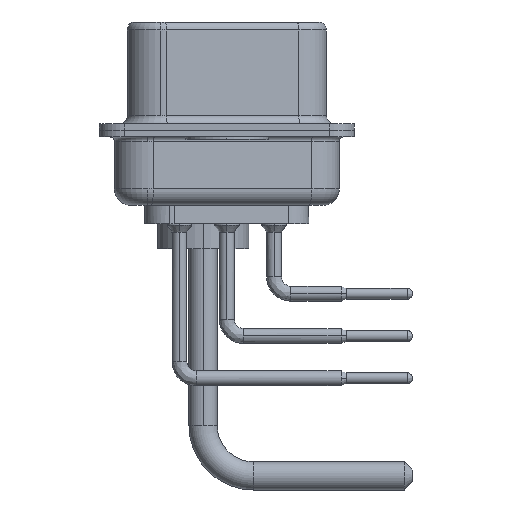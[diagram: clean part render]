
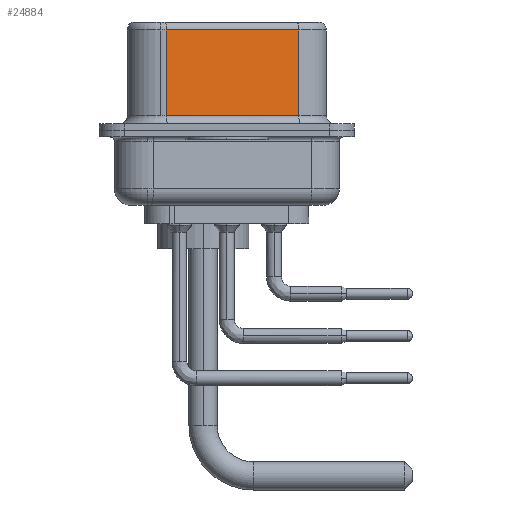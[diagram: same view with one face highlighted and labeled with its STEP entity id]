
A CAD part, left-side view. The second image highlights one B-rep face of the part: STEP entity #24884.
In plain terms, the highlighted planar face has unit normal (-0.985, -0.174, 0).
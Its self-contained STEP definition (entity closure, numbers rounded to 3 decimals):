
#595 = CARTESIAN_POINT ( 'NONE',  ( 5.132, -4.322, 0.9 ) ) ;
#797 = ORIENTED_EDGE ( 'NONE', *, *, #5857, .F. ) ;
#1269 = VERTEX_POINT ( 'NONE', #9438 ) ;
#2183 = ORIENTED_EDGE ( 'NONE', *, *, #24834, .T. ) ;
#3165 = CARTESIAN_POINT ( 'NONE',  ( 3.73, 3.628, 0.9 ) ) ;
#3638 = DIRECTION ( 'NONE',  ( 0., 0., -1. ) ) ;
#4815 = EDGE_CURVE ( 'NONE', #26537, #24399, #20676, .T. ) ;
#5748 = CARTESIAN_POINT ( 'NONE',  ( 5.132, -4.322, 6.02 ) ) ;
#5857 = EDGE_CURVE ( 'NONE', #13186, #24399, #33893, .T. ) ;
#6937 = DIRECTION ( 'NONE',  ( 0., 0., -1. ) ) ;
#9073 = AXIS2_PLACEMENT_3D ( 'NONE', #27571, #14361, #24954 ) ;
#9111 = FACE_OUTER_BOUND ( 'NONE', #25053, .T. ) ;
#9289 = VECTOR ( 'NONE', #18236, 1000. ) ;
#9438 = CARTESIAN_POINT ( 'NONE',  ( 3.73, 3.628, 6.02 ) ) ;
#10069 = ORIENTED_EDGE ( 'NONE', *, *, #4815, .T. ) ;
#12164 = LINE ( 'NONE', #22770, #21083 ) ;
#13186 = VERTEX_POINT ( 'NONE', #5748 ) ;
#13521 = VECTOR ( 'NONE', #29665, 1000. ) ;
#14361 = DIRECTION ( 'NONE',  ( 0.985, 0.174, 0. ) ) ;
#16967 = PLANE ( 'NONE',  #9073 ) ;
#18236 = DIRECTION ( 'NONE',  ( 0.174, -0.985, 0. ) ) ;
#18398 = CARTESIAN_POINT ( 'NONE',  ( 5.132, -4.322, 0.9 ) ) ;
#19882 = EDGE_CURVE ( 'NONE', #1269, #26537, #12164, .T. ) ;
#19922 = VECTOR ( 'NONE', #6937, 1000. ) ;
#20676 = LINE ( 'NONE', #18398, #9289 ) ;
#21083 = VECTOR ( 'NONE', #3638, 1000. ) ;
#21650 = CARTESIAN_POINT ( 'NONE',  ( 5.132, -4.322, 6.02 ) ) ;
#22770 = CARTESIAN_POINT ( 'NONE',  ( 3.73, 3.628, 6.52 ) ) ;
#22779 = CARTESIAN_POINT ( 'NONE',  ( 5.132, -4.322, 6.52 ) ) ;
#23377 = ORIENTED_EDGE ( 'NONE', *, *, #19882, .T. ) ;
#24399 = VERTEX_POINT ( 'NONE', #595 ) ;
#24834 = EDGE_CURVE ( 'NONE', #13186, #1269, #27210, .T. ) ;
#24884 = ADVANCED_FACE ( 'NONE', ( #9111 ), #16967, .F. ) ;
#24954 = DIRECTION ( 'NONE',  ( -0.174, 0.985, 0. ) ) ;
#25053 = EDGE_LOOP ( 'NONE', ( #797, #2183, #23377, #10069 ) ) ;
#26537 = VERTEX_POINT ( 'NONE', #3165 ) ;
#27210 = LINE ( 'NONE', #21650, #13521 ) ;
#27571 = CARTESIAN_POINT ( 'NONE',  ( 5.132, -4.322, 6.52 ) ) ;
#29665 = DIRECTION ( 'NONE',  ( -0.174, 0.985, 0. ) ) ;
#33893 = LINE ( 'NONE', #22779, #19922 ) ;
